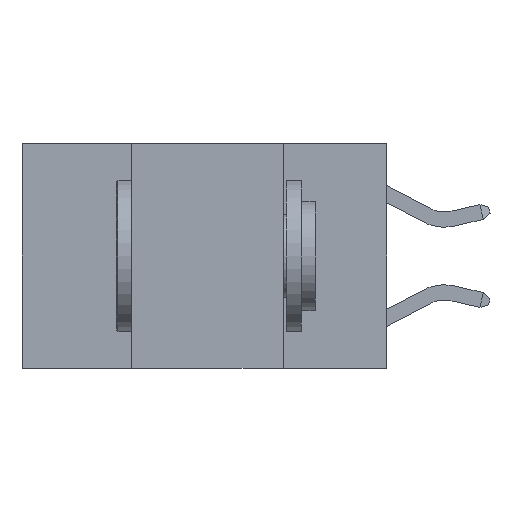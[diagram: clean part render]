
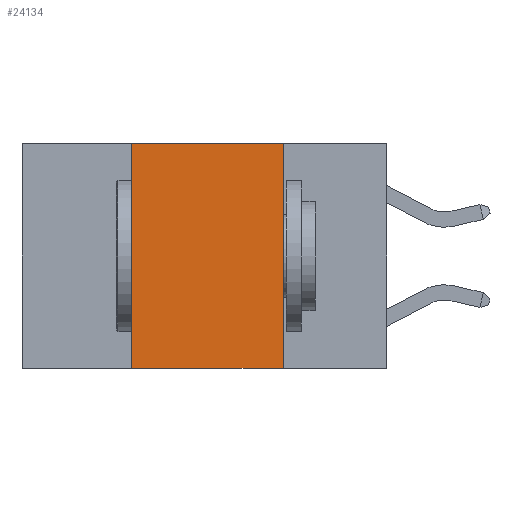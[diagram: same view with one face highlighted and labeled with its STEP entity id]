
A CAD part, left-side view. The second image highlights one B-rep face of the part: STEP entity #24134.
In plain terms, the highlighted planar face has unit normal (-1, 0, 0).
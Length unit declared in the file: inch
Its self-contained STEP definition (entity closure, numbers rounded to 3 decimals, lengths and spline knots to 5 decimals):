
#437 = EDGE_CURVE ( 'NONE', #28242, #28037, #2102, .T. ) ;
#1292 = CARTESIAN_POINT ( 'NONE',  ( 0., 0.42, 0. ) ) ;
#2102 = LINE ( 'NONE', #9691, #7981 ) ;
#3667 = VECTOR ( 'NONE', #23954, 39.37008 ) ;
#4456 = ORIENTED_EDGE ( 'NONE', *, *, #437, .F. ) ;
#5590 = DIRECTION ( 'NONE',  ( 0., 0., 1. ) ) ;
#5896 = LINE ( 'NONE', #1292, #18496 ) ;
#6673 = EDGE_CURVE ( 'NONE', #12962, #28242, #28611, .T. ) ;
#7619 = CARTESIAN_POINT ( 'NONE',  ( 0., 0.42, -0.37 ) ) ;
#7981 = VECTOR ( 'NONE', #19237, 39.37008 ) ;
#8977 = ORIENTED_EDGE ( 'NONE', *, *, #6673, .F. ) ;
#9243 = AXIS2_PLACEMENT_3D ( 'NONE', #16956, #18851, #19307 ) ;
#9691 = CARTESIAN_POINT ( 'NONE',  ( 0., 0.17, 0. ) ) ;
#11020 = EDGE_CURVE ( 'NONE', #23288, #28037, #23795, .T. ) ;
#12962 = VERTEX_POINT ( 'NONE', #18946 ) ;
#14627 = FACE_OUTER_BOUND ( 'NONE', #17678, .T. ) ;
#15094 = ORIENTED_EDGE ( 'NONE', *, *, #11020, .T. ) ;
#16483 = PLANE ( 'NONE',  #9243 ) ;
#16660 = EDGE_CURVE ( 'NONE', #23288, #12962, #5896, .T. ) ;
#16884 = CARTESIAN_POINT ( 'NONE',  ( 0., 0.17, -0.37 ) ) ;
#16956 = CARTESIAN_POINT ( 'NONE',  ( 0., 0.6, 0. ) ) ;
#17678 = EDGE_LOOP ( 'NONE', ( #4456, #8977, #21244, #15094 ) ) ;
#18496 = VECTOR ( 'NONE', #5590, 39.37008 ) ;
#18851 = DIRECTION ( 'NONE',  ( 1., 0., 0. ) ) ;
#18946 = CARTESIAN_POINT ( 'NONE',  ( 0., 0.42, 0. ) ) ;
#19237 = DIRECTION ( 'NONE',  ( 0., 0., -1. ) ) ;
#19307 = DIRECTION ( 'NONE',  ( 0., 0., -1. ) ) ;
#20940 = DIRECTION ( 'NONE',  ( 0., -1., 0. ) ) ;
#21244 = ORIENTED_EDGE ( 'NONE', *, *, #16660, .F. ) ;
#23288 = VERTEX_POINT ( 'NONE', #7619 ) ;
#23795 = LINE ( 'NONE', #28440, #26316 ) ;
#23954 = DIRECTION ( 'NONE',  ( 0., -1., 0. ) ) ;
#24134 = ADVANCED_FACE ( 'NONE', ( #14627 ), #16483, .F. ) ;
#24731 = CARTESIAN_POINT ( 'NONE',  ( 0., 0.17, 0. ) ) ;
#26316 = VECTOR ( 'NONE', #20940, 39.37008 ) ;
#26601 = CARTESIAN_POINT ( 'NONE',  ( 0., 0.6, 0. ) ) ;
#28037 = VERTEX_POINT ( 'NONE', #16884 ) ;
#28242 = VERTEX_POINT ( 'NONE', #24731 ) ;
#28440 = CARTESIAN_POINT ( 'NONE',  ( 0., 0.6, -0.37 ) ) ;
#28611 = LINE ( 'NONE', #26601, #3667 ) ;
